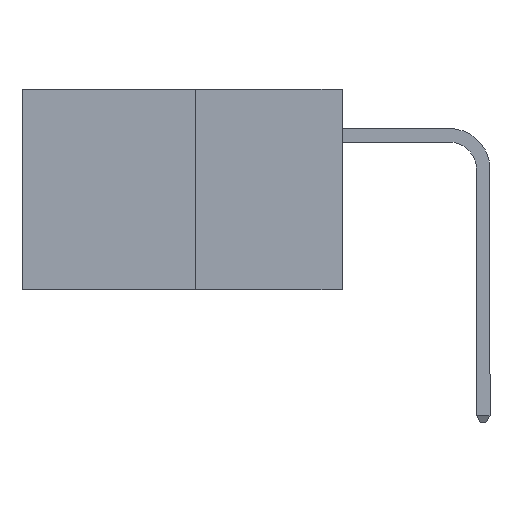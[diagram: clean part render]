
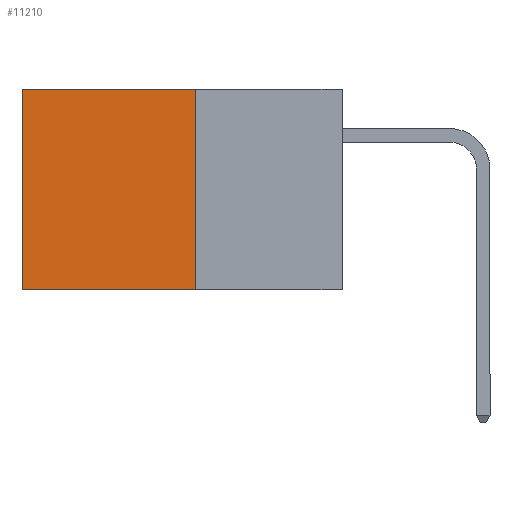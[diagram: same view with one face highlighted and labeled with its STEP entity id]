
A CAD part, left-side view. The second image highlights one B-rep face of the part: STEP entity #11210.
In plain terms, the highlighted planar face has unit normal (-1, 0, 0).
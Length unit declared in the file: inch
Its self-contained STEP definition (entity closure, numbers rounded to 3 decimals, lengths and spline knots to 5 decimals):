
#21 = DIRECTION ( 'NONE',  ( 1., 0., 0. ) ) ;
#44 = VERTEX_POINT ( 'NONE', #304 ) ;
#304 = CARTESIAN_POINT ( 'NONE',  ( 0.277, 0.59, 0. ) ) ;
#523 = VERTEX_POINT ( 'NONE', #8979 ) ;
#557 = VECTOR ( 'NONE', #11690, 39.37008 ) ;
#1307 = CARTESIAN_POINT ( 'NONE',  ( 0.277, 0.27, -0.37 ) ) ;
#1569 = EDGE_LOOP ( 'NONE', ( #11270, #1969, #4398, #11555 ) ) ;
#1825 = VECTOR ( 'NONE', #7396, 39.37008 ) ;
#1907 = VECTOR ( 'NONE', #9219, 39.37008 ) ;
#1969 = ORIENTED_EDGE ( 'NONE', *, *, #5481, .F. ) ;
#2489 = FACE_OUTER_BOUND ( 'NONE', #1569, .T. ) ;
#2512 = AXIS2_PLACEMENT_3D ( 'NONE', #3716, #21, #6479 ) ;
#2859 = CARTESIAN_POINT ( 'NONE',  ( 0.277, 0.27, 0. ) ) ;
#3390 = VERTEX_POINT ( 'NONE', #6933 ) ;
#3716 = CARTESIAN_POINT ( 'NONE',  ( 0.277, 0.27, -0.37 ) ) ;
#4041 = LINE ( 'NONE', #2859, #1907 ) ;
#4398 = ORIENTED_EDGE ( 'NONE', *, *, #8839, .F. ) ;
#4452 = LINE ( 'NONE', #1307, #8997 ) ;
#4657 = CARTESIAN_POINT ( 'NONE',  ( 0.277, 0.27, -0.37 ) ) ;
#5481 = EDGE_CURVE ( 'NONE', #7816, #523, #11410, .T. ) ;
#5839 = DIRECTION ( 'NONE',  ( 0., 0., -1. ) ) ;
#6032 = LINE ( 'NONE', #8112, #557 ) ;
#6479 = DIRECTION ( 'NONE',  ( 0., 0., -1. ) ) ;
#6933 = CARTESIAN_POINT ( 'NONE',  ( 0.277, 0.27, 0. ) ) ;
#7338 = PLANE ( 'NONE',  #2512 ) ;
#7396 = DIRECTION ( 'NONE',  ( 0., 1., 0. ) ) ;
#7816 = VERTEX_POINT ( 'NONE', #10832 ) ;
#7887 = EDGE_CURVE ( 'NONE', #3390, #44, #4041, .T. ) ;
#8112 = CARTESIAN_POINT ( 'NONE',  ( 0.277, 0.59, -0.37 ) ) ;
#8839 = EDGE_CURVE ( 'NONE', #3390, #7816, #4452, .T. ) ;
#8979 = CARTESIAN_POINT ( 'NONE',  ( 0.277, 0.59, -0.37 ) ) ;
#8997 = VECTOR ( 'NONE', #5839, 39.37008 ) ;
#9201 = EDGE_CURVE ( 'NONE', #44, #523, #6032, .T. ) ;
#9219 = DIRECTION ( 'NONE',  ( 0., 1., 0. ) ) ;
#10832 = CARTESIAN_POINT ( 'NONE',  ( 0.277, 0.27, -0.37 ) ) ;
#11210 = ADVANCED_FACE ( 'NONE', ( #2489 ), #7338, .F. ) ;
#11270 = ORIENTED_EDGE ( 'NONE', *, *, #9201, .T. ) ;
#11410 = LINE ( 'NONE', #4657, #1825 ) ;
#11555 = ORIENTED_EDGE ( 'NONE', *, *, #7887, .T. ) ;
#11690 = DIRECTION ( 'NONE',  ( 0., 0., -1. ) ) ;
